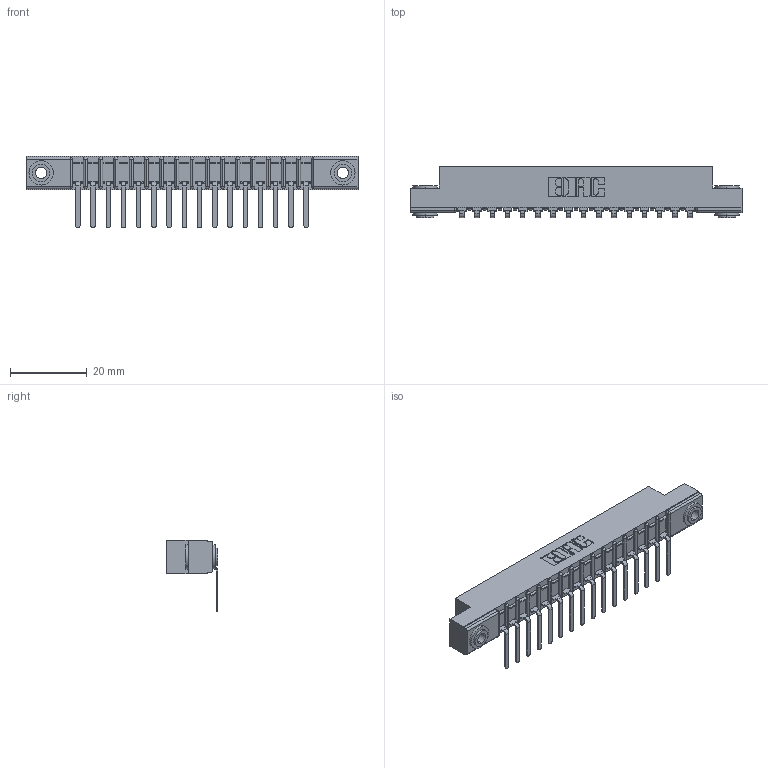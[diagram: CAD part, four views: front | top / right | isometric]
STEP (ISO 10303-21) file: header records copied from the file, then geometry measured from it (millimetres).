
FILE_DESCRIPTION (( 'STEP AP203' ), '1' );
FILE_NAME ('307-016-557-103.STEP', '2018-08-03T03:34:30', ( '' ), ( '' ), 'SwSTEP 2.0', 'SolidWorks 2016', '' );
FILE_SCHEMA (( 'CONFIG_CONTROL_DESIGN' ));
Length unit declared in the file: inch
Products named in the file (4): 345-250-002_345-250-002-102; 307-016-557-103; 307 Part_.156 Dia Mounting Holes; 307-290-002_557
Assembly tree (19 placements, depth 2):
  307-016-557-103
    307 Part_.156 Dia Mounting Holes
    307-290-002_557  x16
    345-250-002_345-250-002-102  x2
Bounding box: 86.41 x 13.36 x 18.67 mm (x, y, z)
Volume: 5746 mm3; surface area: 10625.2 mm2
Topology: 19 solids, 19 shells, 1435 faces, 4339 edges, 2842 vertices
Faces by surface type: plane 846, cylinder 547, sphere 34, cone 8
Entity records: 18841 total; most frequent: CARTESIAN_POINT 3153, ORIENTED_EDGE 3134, DIRECTION 3091, EDGE_CURVE 1567, VECTOR 1179, LINE 1179, VERTEX_POINT 1018, AXIS2_PLACEMENT_3D 956
